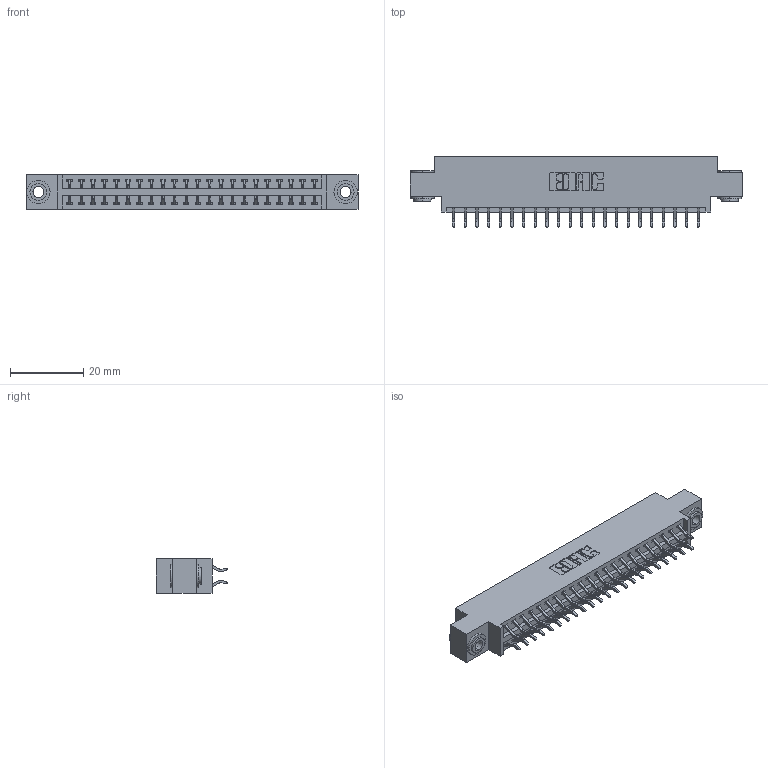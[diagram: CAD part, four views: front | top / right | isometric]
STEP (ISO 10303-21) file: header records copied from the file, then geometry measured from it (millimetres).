
FILE_DESCRIPTION (( 'STEP AP203' ), '1' );
FILE_NAME ('396-044-556-803.STEP', '2019-11-02T06:29:52', ( '' ), ( '' ), 'SwSTEP 2.0', 'SolidWorks 2016', '' );
FILE_SCHEMA (( 'CONFIG_CONTROL_DESIGN' ));
Length unit declared in the file: inch
Products named in the file (4): 346 Part_0.170 Offset - 0.156 Dia-TH; 345-292-001_556 Tail; 345-250-002_345-250-002-102; 396-044-556-803
Assembly tree (47 placements, depth 2):
  396-044-556-803
    346 Part_0.170 Offset - 0.156 Dia-TH
    345-292-001_556 Tail  x44
    345-250-002_345-250-002-102  x2
Bounding box: 90.42 x 19.57 x 9.4 mm (x, y, z)
Volume: 8525.2 mm3; surface area: 11757 mm2
Topology: 47 solids, 47 shells, 2716 faces, 8029 edges, 5290 vertices
Faces by surface type: plane 1806, cylinder 902, cone 8
Entity records: 18052 total; most frequent: CARTESIAN_POINT 2995, ORIENTED_EDGE 2910, DIRECTION 2709, EDGE_CURVE 1455, VECTOR 1203, LINE 1203, VERTEX_POINT 966, AXIS2_PLACEMENT_3D 753
